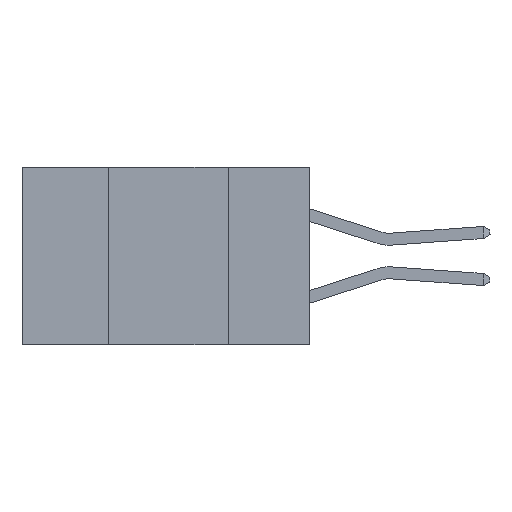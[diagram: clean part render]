
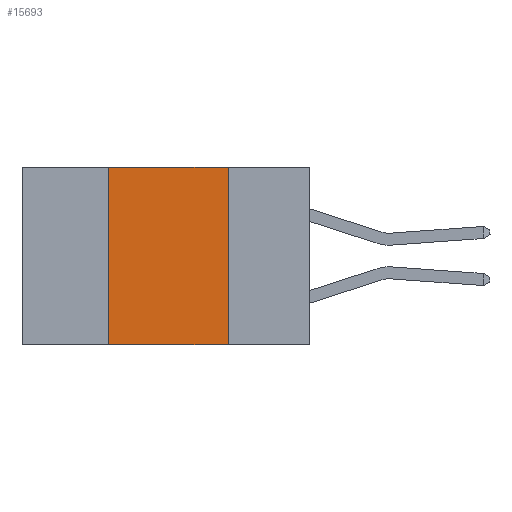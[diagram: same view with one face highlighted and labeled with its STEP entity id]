
A CAD part, left-side view. The second image highlights one B-rep face of the part: STEP entity #15693.
In plain terms, the highlighted planar face has unit normal (-1, 0, 0).
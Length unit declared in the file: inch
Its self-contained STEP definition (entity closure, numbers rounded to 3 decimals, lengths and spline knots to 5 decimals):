
#669 = CARTESIAN_POINT ( 'NONE',  ( 0., 0.42, 0. ) ) ;
#745 = VERTEX_POINT ( 'NONE', #25305 ) ;
#1073 = LINE ( 'NONE', #26530, #25264 ) ;
#2695 = PLANE ( 'NONE',  #13362 ) ;
#2712 = VECTOR ( 'NONE', #11395, 39.37008 ) ;
#4734 = VECTOR ( 'NONE', #14325, 39.37008 ) ;
#5161 = VECTOR ( 'NONE', #13245, 39.37008 ) ;
#9143 = CARTESIAN_POINT ( 'NONE',  ( 0., 0.42, -0.37 ) ) ;
#10116 = EDGE_CURVE ( 'NONE', #17992, #26682, #1073, .T. ) ;
#10232 = DIRECTION ( 'NONE',  ( 0., -1., 0. ) ) ;
#10935 = LINE ( 'NONE', #11963, #4734 ) ;
#11140 = EDGE_LOOP ( 'NONE', ( #13098, #14545, #17885, #26977 ) ) ;
#11377 = VERTEX_POINT ( 'NONE', #9143 ) ;
#11395 = DIRECTION ( 'NONE',  ( 0., 0., -1. ) ) ;
#11963 = CARTESIAN_POINT ( 'NONE',  ( 0., 0.6, -0.37 ) ) ;
#12084 = DIRECTION ( 'NONE',  ( 1., 0., 0. ) ) ;
#12750 = EDGE_CURVE ( 'NONE', #26682, #745, #14423, .T. ) ;
#13098 = ORIENTED_EDGE ( 'NONE', *, *, #12750, .F. ) ;
#13142 = CARTESIAN_POINT ( 'NONE',  ( 0., 0.42, 0. ) ) ;
#13245 = DIRECTION ( 'NONE',  ( 0., 0., 1. ) ) ;
#13362 = AXIS2_PLACEMENT_3D ( 'NONE', #26141, #12084, #28446 ) ;
#14325 = DIRECTION ( 'NONE',  ( 0., -1., 0. ) ) ;
#14423 = LINE ( 'NONE', #23119, #2712 ) ;
#14545 = ORIENTED_EDGE ( 'NONE', *, *, #10116, .F. ) ;
#15693 = ADVANCED_FACE ( 'NONE', ( #21541 ), #2695, .F. ) ;
#17885 = ORIENTED_EDGE ( 'NONE', *, *, #20174, .F. ) ;
#17992 = VERTEX_POINT ( 'NONE', #669 ) ;
#20174 = EDGE_CURVE ( 'NONE', #11377, #17992, #23886, .T. ) ;
#21541 = FACE_OUTER_BOUND ( 'NONE', #11140, .T. ) ;
#23119 = CARTESIAN_POINT ( 'NONE',  ( 0., 0.17, 0. ) ) ;
#23886 = LINE ( 'NONE', #13142, #5161 ) ;
#24301 = CARTESIAN_POINT ( 'NONE',  ( 0., 0.17, 0. ) ) ;
#25264 = VECTOR ( 'NONE', #10232, 39.37008 ) ;
#25305 = CARTESIAN_POINT ( 'NONE',  ( 0., 0.17, -0.37 ) ) ;
#26141 = CARTESIAN_POINT ( 'NONE',  ( 0., 0.6, 0. ) ) ;
#26530 = CARTESIAN_POINT ( 'NONE',  ( 0., 0.6, 0. ) ) ;
#26682 = VERTEX_POINT ( 'NONE', #24301 ) ;
#26977 = ORIENTED_EDGE ( 'NONE', *, *, #28594, .T. ) ;
#28446 = DIRECTION ( 'NONE',  ( 0., 0., -1. ) ) ;
#28594 = EDGE_CURVE ( 'NONE', #11377, #745, #10935, .T. ) ;
